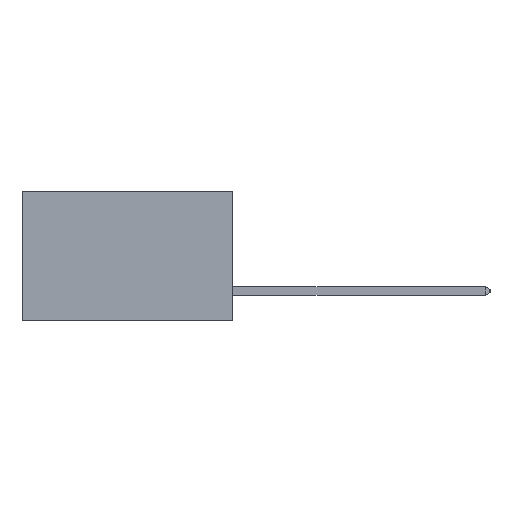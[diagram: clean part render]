
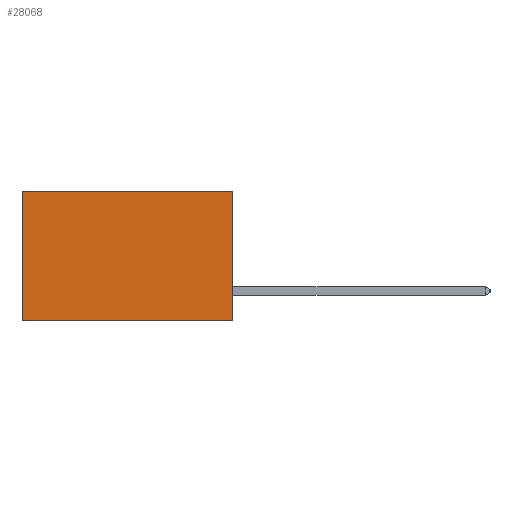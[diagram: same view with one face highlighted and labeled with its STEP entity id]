
A CAD part, left-side view. The second image highlights one B-rep face of the part: STEP entity #28068.
In plain terms, the highlighted planar face has unit normal (-1, 0, 0).
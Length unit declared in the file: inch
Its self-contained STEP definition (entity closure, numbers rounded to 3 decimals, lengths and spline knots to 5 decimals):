
#46 = VERTEX_POINT ( 'NONE', #8991 ) ;
#79 = CARTESIAN_POINT ( 'NONE',  ( 0.2875, 0.6, -0.37 ) ) ;
#909 = VECTOR ( 'NONE', #23137, 39.37008 ) ;
#1003 = EDGE_CURVE ( 'NONE', #12467, #19426, #20245, .T. ) ;
#2808 = EDGE_CURVE ( 'NONE', #46, #12467, #26432, .T. ) ;
#4000 = DIRECTION ( 'NONE',  ( 1., 0., 0. ) ) ;
#5065 = EDGE_CURVE ( 'NONE', #10591, #19426, #24597, .T. ) ;
#6542 = CARTESIAN_POINT ( 'NONE',  ( 0.2875, 0.6, 0. ) ) ;
#6684 = CARTESIAN_POINT ( 'NONE',  ( 0.2875, 0.6, 0. ) ) ;
#7381 = CARTESIAN_POINT ( 'NONE',  ( 0.2875, 0., 0. ) ) ;
#7523 = DIRECTION ( 'NONE',  ( 0., 1., 0. ) ) ;
#8991 = CARTESIAN_POINT ( 'NONE',  ( 0.2875, 0., 0. ) ) ;
#10591 = VERTEX_POINT ( 'NONE', #6684 ) ;
#10863 = DIRECTION ( 'NONE',  ( 0., 1., 0. ) ) ;
#12467 = VERTEX_POINT ( 'NONE', #26951 ) ;
#12567 = LINE ( 'NONE', #26241, #24900 ) ;
#12938 = CARTESIAN_POINT ( 'NONE',  ( 0.2875, 0., 0. ) ) ;
#15112 = VECTOR ( 'NONE', #7523, 39.37008 ) ;
#16749 = DIRECTION ( 'NONE',  ( 0., 0., -1. ) ) ;
#17192 = AXIS2_PLACEMENT_3D ( 'NONE', #12938, #4000, #19484 ) ;
#19426 = VERTEX_POINT ( 'NONE', #79 ) ;
#19484 = DIRECTION ( 'NONE',  ( 0., 0., -1. ) ) ;
#19830 = VECTOR ( 'NONE', #16749, 39.37008 ) ;
#20245 = LINE ( 'NONE', #28105, #15112 ) ;
#21953 = ORIENTED_EDGE ( 'NONE', *, *, #1003, .F. ) ;
#22037 = FACE_OUTER_BOUND ( 'NONE', #28444, .T. ) ;
#22392 = ORIENTED_EDGE ( 'NONE', *, *, #26714, .T. ) ;
#23137 = DIRECTION ( 'NONE',  ( 0., 0., -1. ) ) ;
#23849 = PLANE ( 'NONE',  #17192 ) ;
#24597 = LINE ( 'NONE', #6542, #909 ) ;
#24900 = VECTOR ( 'NONE', #10863, 39.37008 ) ;
#25123 = ORIENTED_EDGE ( 'NONE', *, *, #5065, .T. ) ;
#26096 = ORIENTED_EDGE ( 'NONE', *, *, #2808, .F. ) ;
#26241 = CARTESIAN_POINT ( 'NONE',  ( 0.2875, 0., 0. ) ) ;
#26432 = LINE ( 'NONE', #7381, #19830 ) ;
#26714 = EDGE_CURVE ( 'NONE', #46, #10591, #12567, .T. ) ;
#26951 = CARTESIAN_POINT ( 'NONE',  ( 0.2875, 0., -0.37 ) ) ;
#28068 = ADVANCED_FACE ( 'NONE', ( #22037 ), #23849, .F. ) ;
#28105 = CARTESIAN_POINT ( 'NONE',  ( 0.2875, 0., -0.37 ) ) ;
#28444 = EDGE_LOOP ( 'NONE', ( #25123, #21953, #26096, #22392 ) ) ;
